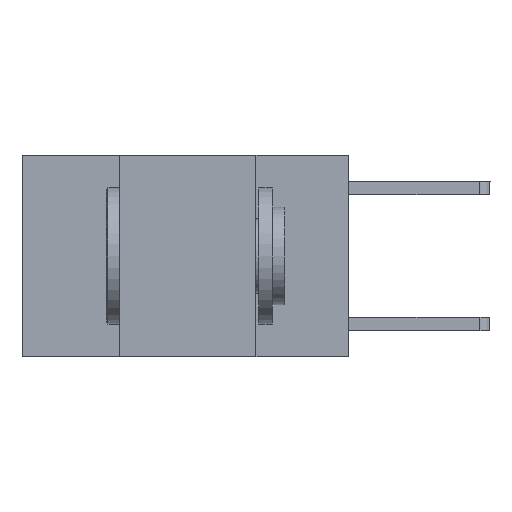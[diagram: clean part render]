
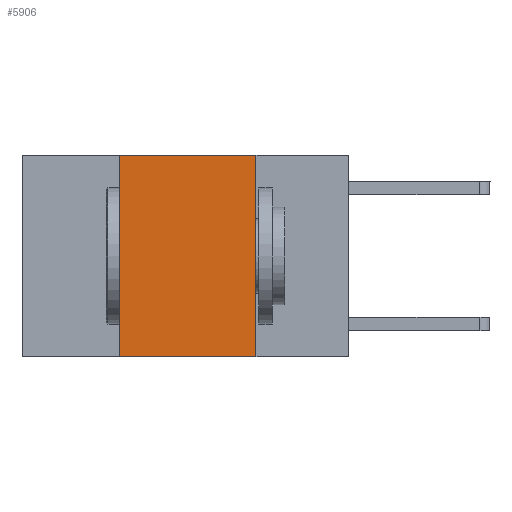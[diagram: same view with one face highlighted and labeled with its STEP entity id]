
A CAD part, left-side view. The second image highlights one B-rep face of the part: STEP entity #5906.
In plain terms, the highlighted planar face has unit normal (-1, 0, 0).
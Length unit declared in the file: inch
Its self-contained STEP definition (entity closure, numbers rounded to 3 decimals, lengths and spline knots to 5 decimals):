
#316 = CARTESIAN_POINT ( 'NONE',  ( 0., 0.17, 0. ) ) ;
#565 = VECTOR ( 'NONE', #7079, 39.37008 ) ;
#643 = ORIENTED_EDGE ( 'NONE', *, *, #4819, .F. ) ;
#680 = CARTESIAN_POINT ( 'NONE',  ( 0., 0.17, -0.37 ) ) ;
#1022 = VERTEX_POINT ( 'NONE', #3843 ) ;
#1289 = EDGE_CURVE ( 'NONE', #2715, #1628, #8610, .T. ) ;
#1384 = DIRECTION ( 'NONE',  ( 0., 0., 1. ) ) ;
#1431 = CARTESIAN_POINT ( 'NONE',  ( 0., 0.42, 0. ) ) ;
#1628 = VERTEX_POINT ( 'NONE', #680 ) ;
#1675 = DIRECTION ( 'NONE',  ( 0., 0., -1. ) ) ;
#1929 = EDGE_CURVE ( 'NONE', #5016, #1022, #4839, .T. ) ;
#2575 = EDGE_LOOP ( 'NONE', ( #8113, #643, #8895, #6728 ) ) ;
#2654 = DIRECTION ( 'NONE',  ( 0., -1., 0. ) ) ;
#2715 = VERTEX_POINT ( 'NONE', #316 ) ;
#3173 = CARTESIAN_POINT ( 'NONE',  ( 0., 0.6, 0. ) ) ;
#3262 = VECTOR ( 'NONE', #3983, 39.37008 ) ;
#3374 = VECTOR ( 'NONE', #2654, 39.37008 ) ;
#3843 = CARTESIAN_POINT ( 'NONE',  ( 0., 0.42, 0. ) ) ;
#3983 = DIRECTION ( 'NONE',  ( 0., -1., 0. ) ) ;
#4819 = EDGE_CURVE ( 'NONE', #1022, #2715, #9241, .T. ) ;
#4839 = LINE ( 'NONE', #1431, #6465 ) ;
#5016 = VERTEX_POINT ( 'NONE', #7993 ) ;
#5303 = AXIS2_PLACEMENT_3D ( 'NONE', #9242, #6449, #1675 ) ;
#5906 = ADVANCED_FACE ( 'NONE', ( #6493 ), #6422, .F. ) ;
#5971 = EDGE_CURVE ( 'NONE', #5016, #1628, #7497, .T. ) ;
#6422 = PLANE ( 'NONE',  #5303 ) ;
#6449 = DIRECTION ( 'NONE',  ( 1., 0., 0. ) ) ;
#6465 = VECTOR ( 'NONE', #1384, 39.37008 ) ;
#6493 = FACE_OUTER_BOUND ( 'NONE', #2575, .T. ) ;
#6728 = ORIENTED_EDGE ( 'NONE', *, *, #5971, .T. ) ;
#7079 = DIRECTION ( 'NONE',  ( 0., 0., -1. ) ) ;
#7314 = CARTESIAN_POINT ( 'NONE',  ( 0., 0.6, -0.37 ) ) ;
#7497 = LINE ( 'NONE', #7314, #3374 ) ;
#7695 = CARTESIAN_POINT ( 'NONE',  ( 0., 0.17, 0. ) ) ;
#7993 = CARTESIAN_POINT ( 'NONE',  ( 0., 0.42, -0.37 ) ) ;
#8113 = ORIENTED_EDGE ( 'NONE', *, *, #1289, .F. ) ;
#8610 = LINE ( 'NONE', #7695, #565 ) ;
#8895 = ORIENTED_EDGE ( 'NONE', *, *, #1929, .F. ) ;
#9241 = LINE ( 'NONE', #3173, #3262 ) ;
#9242 = CARTESIAN_POINT ( 'NONE',  ( 0., 0.6, 0. ) ) ;
